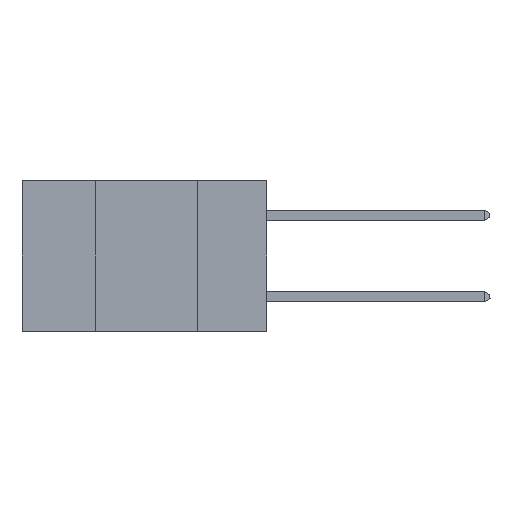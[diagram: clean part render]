
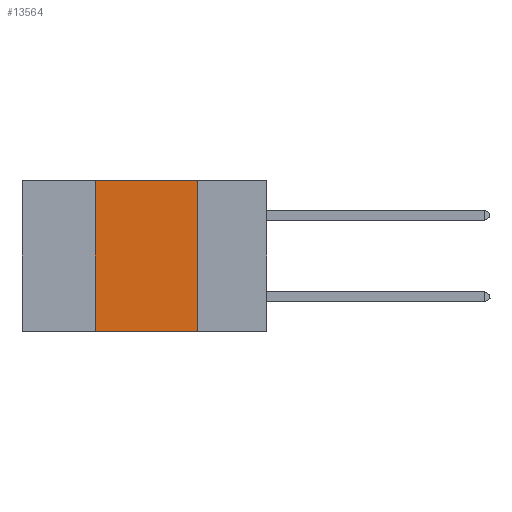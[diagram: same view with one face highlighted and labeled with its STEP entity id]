
A CAD part, left-side view. The second image highlights one B-rep face of the part: STEP entity #13564.
In plain terms, the highlighted planar face has unit normal (-1, 0, 0).
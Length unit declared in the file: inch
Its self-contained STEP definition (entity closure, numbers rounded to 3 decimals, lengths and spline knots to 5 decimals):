
#454 = DIRECTION ( 'NONE',  ( 0., 0., -1. ) ) ;
#1338 = ORIENTED_EDGE ( 'NONE', *, *, #14958, .F. ) ;
#1489 = VERTEX_POINT ( 'NONE', #8782 ) ;
#1582 = PLANE ( 'NONE',  #4498 ) ;
#2220 = LINE ( 'NONE', #2778, #14515 ) ;
#2629 = DIRECTION ( 'NONE',  ( 0., -1., 0. ) ) ;
#2743 = FACE_OUTER_BOUND ( 'NONE', #3889, .T. ) ;
#2778 = CARTESIAN_POINT ( 'NONE',  ( 0., 0.6, 0. ) ) ;
#3425 = DIRECTION ( 'NONE',  ( 0., 0., -1. ) ) ;
#3889 = EDGE_LOOP ( 'NONE', ( #1338, #4804, #13299, #13324 ) ) ;
#4386 = VECTOR ( 'NONE', #9524, 39.37008 ) ;
#4498 = AXIS2_PLACEMENT_3D ( 'NONE', #9920, #5272, #454 ) ;
#4804 = ORIENTED_EDGE ( 'NONE', *, *, #7176, .F. ) ;
#5200 = VERTEX_POINT ( 'NONE', #8971 ) ;
#5261 = CARTESIAN_POINT ( 'NONE',  ( 0., 0.6, -0.37 ) ) ;
#5272 = DIRECTION ( 'NONE',  ( 1., 0., 0. ) ) ;
#6068 = VECTOR ( 'NONE', #14784, 39.37008 ) ;
#6791 = VECTOR ( 'NONE', #3425, 39.37008 ) ;
#7176 = EDGE_CURVE ( 'NONE', #14185, #5200, #2220, .T. ) ;
#7712 = LINE ( 'NONE', #15389, #6791 ) ;
#7746 = LINE ( 'NONE', #5261, #6068 ) ;
#8640 = LINE ( 'NONE', #14657, #4386 ) ;
#8782 = CARTESIAN_POINT ( 'NONE',  ( 0., 0.17, -0.37 ) ) ;
#8971 = CARTESIAN_POINT ( 'NONE',  ( 0., 0.17, 0. ) ) ;
#9045 = EDGE_CURVE ( 'NONE', #14008, #14185, #8640, .T. ) ;
#9524 = DIRECTION ( 'NONE',  ( 0., 0., 1. ) ) ;
#9920 = CARTESIAN_POINT ( 'NONE',  ( 0., 0.6, 0. ) ) ;
#12559 = CARTESIAN_POINT ( 'NONE',  ( 0., 0.42, 0. ) ) ;
#13299 = ORIENTED_EDGE ( 'NONE', *, *, #9045, .F. ) ;
#13324 = ORIENTED_EDGE ( 'NONE', *, *, #14056, .T. ) ;
#13564 = ADVANCED_FACE ( 'NONE', ( #2743 ), #1582, .F. ) ;
#13658 = CARTESIAN_POINT ( 'NONE',  ( 0., 0.42, -0.37 ) ) ;
#14008 = VERTEX_POINT ( 'NONE', #13658 ) ;
#14056 = EDGE_CURVE ( 'NONE', #14008, #1489, #7746, .T. ) ;
#14185 = VERTEX_POINT ( 'NONE', #12559 ) ;
#14515 = VECTOR ( 'NONE', #2629, 39.37008 ) ;
#14657 = CARTESIAN_POINT ( 'NONE',  ( 0., 0.42, 0. ) ) ;
#14784 = DIRECTION ( 'NONE',  ( 0., -1., 0. ) ) ;
#14958 = EDGE_CURVE ( 'NONE', #5200, #1489, #7712, .T. ) ;
#15389 = CARTESIAN_POINT ( 'NONE',  ( 0., 0.17, 0. ) ) ;
